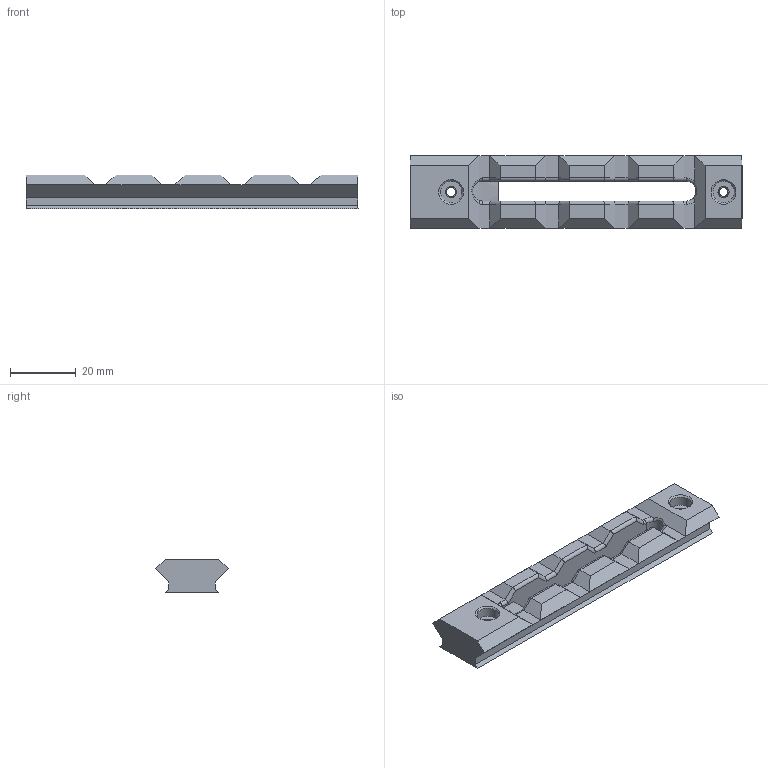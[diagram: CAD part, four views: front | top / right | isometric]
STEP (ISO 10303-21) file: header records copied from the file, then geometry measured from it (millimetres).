
FILE_DESCRIPTION (( 'STEP AP203' ), '1' );
FILE_NAME ('side_rail.STEP', '2020-05-10T05:52:13', ( '' ), ( '' ), 'SwSTEP 2.0', 'SolidWorks 2016', '' );
FILE_SCHEMA (( 'CONFIG_CONTROL_DESIGN' ));
Length unit declared in the file: millimetre
Products named in the file (1): side_rail
Bounding box: 100.82 x 22.05 x 10.28 mm (x, y, z)
Volume: 12559.9 mm3; surface area: 7112 mm2
Topology: 1 solids, 1 shells, 99 faces, 238 edges, 144 vertices
Faces by surface type: plane 56, cylinder 35, torus 4, cone 2, bspline 2
Full cylindrical faces by diameter (mm): 2.7 x2, 3.4 x2, 6.5 x2
Entity records: 3061 total; most frequent: CARTESIAN_POINT 819, ORIENTED_EDGE 456, DIRECTION 415, EDGE_CURVE 228, LINE 163, VECTOR 163, VERTEX_POINT 142, AXIS2_PLACEMENT_3D 126
